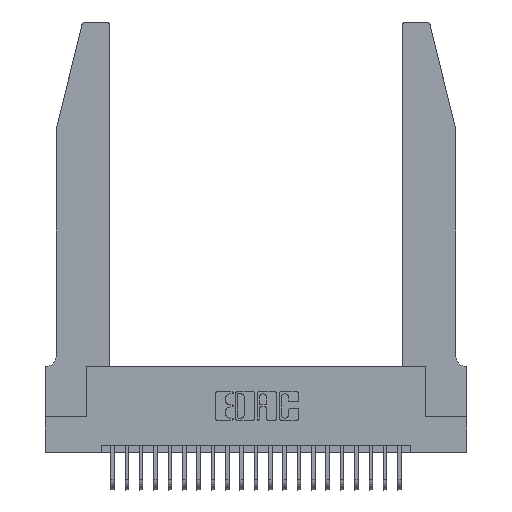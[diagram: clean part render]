
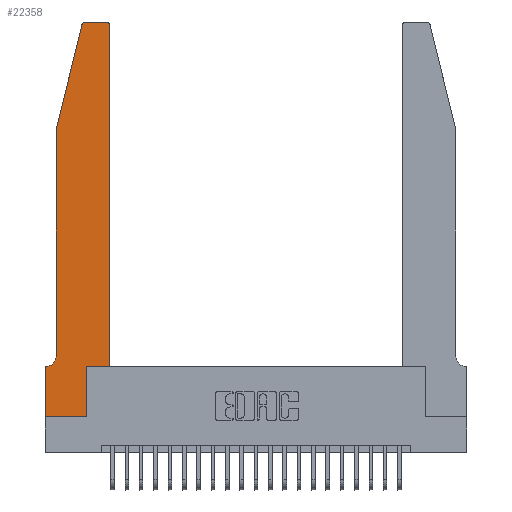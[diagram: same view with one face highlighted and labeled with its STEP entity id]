
A CAD part, top view. The second image highlights one B-rep face of the part: STEP entity #22358.
In plain terms, the highlighted planar face has unit normal (0, 0, 1).
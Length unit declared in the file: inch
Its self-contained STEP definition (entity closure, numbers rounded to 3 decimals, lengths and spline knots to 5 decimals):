
#276 = CARTESIAN_POINT ( 'NONE',  ( 0.4505, 2.72, 0.37 ) ) ;
#398 = DIRECTION ( 'NONE',  ( 1., 0., 0. ) ) ;
#477 = VERTEX_POINT ( 'NONE', #276 ) ;
#687 = AXIS2_PLACEMENT_3D ( 'NONE', #13670, #1573, #15613 ) ;
#795 = LINE ( 'NONE', #8910, #11031 ) ;
#949 = ORIENTED_EDGE ( 'NONE', *, *, #25174, .T. ) ;
#1255 = DIRECTION ( 'NONE',  ( 0., 1., 0. ) ) ;
#1522 = VECTOR ( 'NONE', #4026, 39.37008 ) ;
#1573 = DIRECTION ( 'NONE',  ( 0., 0., 1. ) ) ;
#1868 = VERTEX_POINT ( 'NONE', #6498 ) ;
#1920 = VERTEX_POINT ( 'NONE', #20154 ) ;
#1921 = CARTESIAN_POINT ( 'NONE',  ( 0.0755, 2., 0.37 ) ) ;
#2319 = AXIS2_PLACEMENT_3D ( 'NONE', #24216, #12634, #398 ) ;
#2850 = CIRCLE ( 'NONE', #23031, 0.07 ) ;
#3149 = CIRCLE ( 'NONE', #12000, 0.03 ) ;
#3510 = CARTESIAN_POINT ( 'NONE',  ( 0.2865, 0., 0.37 ) ) ;
#3579 = CARTESIAN_POINT ( 'NONE',  ( 0.0055, 0.42, 0.37 ) ) ;
#3863 = DIRECTION ( 'NONE',  ( 1., 0., 0. ) ) ;
#4026 = DIRECTION ( 'NONE',  ( 1., 0., 0. ) ) ;
#4097 = VERTEX_POINT ( 'NONE', #22387 ) ;
#4926 = ORIENTED_EDGE ( 'NONE', *, *, #16400, .T. ) ;
#5160 = VERTEX_POINT ( 'NONE', #10495 ) ;
#5360 = CARTESIAN_POINT ( 'NONE',  ( 0.2605, 2.75, 0.37 ) ) ;
#5563 = ORIENTED_EDGE ( 'NONE', *, *, #16069, .T. ) ;
#5650 = DIRECTION ( 'NONE',  ( -1., 0., 0. ) ) ;
#6498 = CARTESIAN_POINT ( 'NONE',  ( 0.25487, 2.72718, 0.37 ) ) ;
#6994 = LINE ( 'NONE', #19590, #16216 ) ;
#7205 = CARTESIAN_POINT ( 'NONE',  ( 0., 0., 0.37 ) ) ;
#7231 = VECTOR ( 'NONE', #9652, 39.37008 ) ;
#7433 = DIRECTION ( 'NONE',  ( -1., 0., 0. ) ) ;
#7659 = CARTESIAN_POINT ( 'NONE',  ( 0.2865, 0.35, 0.37 ) ) ;
#7938 = CARTESIAN_POINT ( 'NONE',  ( 0., 0., 0.37 ) ) ;
#7959 = VERTEX_POINT ( 'NONE', #14948 ) ;
#8149 = VERTEX_POINT ( 'NONE', #17433 ) ;
#8910 = CARTESIAN_POINT ( 'NONE',  ( 0.0755, 2., 0.37 ) ) ;
#8956 = LINE ( 'NONE', #13859, #18140 ) ;
#9561 = EDGE_CURVE ( 'NONE', #1920, #19440, #24381, .T. ) ;
#9652 = DIRECTION ( 'NONE',  ( 0., 1., 0. ) ) ;
#9710 = VECTOR ( 'NONE', #1255, 39.37008 ) ;
#9889 = DIRECTION ( 'NONE',  ( -1., 0., 0. ) ) ;
#10101 = VECTOR ( 'NONE', #19632, 39.37008 ) ;
#10132 = EDGE_LOOP ( 'NONE', ( #23525, #24363, #21272, #4926, #16394, #23688, #21248, #5563, #949, #20915, #19216, #16464 ) ) ;
#10495 = CARTESIAN_POINT ( 'NONE',  ( 0.0755, 0.42, 0.37 ) ) ;
#10695 = EDGE_CURVE ( 'NONE', #8149, #17127, #20692, .T. ) ;
#10889 = CARTESIAN_POINT ( 'NONE',  ( 0.4205, 2.72, 0.37 ) ) ;
#10891 = DIRECTION ( 'NONE',  ( 0., -1., 0. ) ) ;
#10953 = VECTOR ( 'NONE', #7433, 39.37008 ) ;
#11031 = VECTOR ( 'NONE', #10891, 39.37008 ) ;
#11214 = EDGE_CURVE ( 'NONE', #15154, #477, #14879, .T. ) ;
#11569 = EDGE_CURVE ( 'NONE', #17127, #1868, #17948, .T. ) ;
#12000 = AXIS2_PLACEMENT_3D ( 'NONE', #10889, #24470, #12870 ) ;
#12634 = DIRECTION ( 'NONE',  ( 0., 0., 1. ) ) ;
#12870 = DIRECTION ( 'NONE',  ( 1., 0., 0. ) ) ;
#13045 = VERTEX_POINT ( 'NONE', #3510 ) ;
#13189 = VERTEX_POINT ( 'NONE', #1921 ) ;
#13670 = CARTESIAN_POINT ( 'NONE',  ( 0., 0.35, 0.37 ) ) ;
#13804 = LINE ( 'NONE', #15768, #23543 ) ;
#13859 = CARTESIAN_POINT ( 'NONE',  ( 0.0755, 2., 0.37 ) ) ;
#14879 = LINE ( 'NONE', #23084, #9710 ) ;
#14927 = EDGE_CURVE ( 'NONE', #1868, #13189, #8956, .T. ) ;
#14948 = CARTESIAN_POINT ( 'NONE',  ( 0.0055, 0.35, 0.37 ) ) ;
#15154 = VERTEX_POINT ( 'NONE', #20471 ) ;
#15613 = DIRECTION ( 'NONE',  ( 1., 0., 0. ) ) ;
#15768 = CARTESIAN_POINT ( 'NONE',  ( 0., 0., 0.37 ) ) ;
#15823 = DIRECTION ( 'NONE',  ( -0.239, -0.971, 0. ) ) ;
#15932 = CARTESIAN_POINT ( 'NONE',  ( 0.4505, 0.35, 0.37 ) ) ;
#16069 = EDGE_CURVE ( 'NONE', #19440, #13045, #13804, .T. ) ;
#16216 = VECTOR ( 'NONE', #9889, 39.37008 ) ;
#16340 = CARTESIAN_POINT ( 'NONE',  ( 0.284, 2.75, 0.37 ) ) ;
#16394 = ORIENTED_EDGE ( 'NONE', *, *, #22010, .T. ) ;
#16400 = EDGE_CURVE ( 'NONE', #13189, #5160, #795, .T. ) ;
#16464 = ORIENTED_EDGE ( 'NONE', *, *, #23301, .T. ) ;
#17127 = VERTEX_POINT ( 'NONE', #16340 ) ;
#17433 = CARTESIAN_POINT ( 'NONE',  ( 0.4205, 2.75, 0.37 ) ) ;
#17469 = DIRECTION ( 'NONE',  ( 0., 0., -1. ) ) ;
#17948 = CIRCLE ( 'NONE', #2319, 0.03 ) ;
#18140 = VECTOR ( 'NONE', #15823, 39.37008 ) ;
#19216 = ORIENTED_EDGE ( 'NONE', *, *, #11214, .T. ) ;
#19440 = VERTEX_POINT ( 'NONE', #7205 ) ;
#19590 = CARTESIAN_POINT ( 'NONE',  ( 0.0755, 0.35, 0.37 ) ) ;
#19632 = DIRECTION ( 'NONE',  ( 0., -1., 0. ) ) ;
#20154 = CARTESIAN_POINT ( 'NONE',  ( 0., 0.35, 0.37 ) ) ;
#20471 = CARTESIAN_POINT ( 'NONE',  ( 0.4505, 0.35, 0.37 ) ) ;
#20692 = LINE ( 'NONE', #5360, #10953 ) ;
#20915 = ORIENTED_EDGE ( 'NONE', *, *, #22157, .T. ) ;
#21248 = ORIENTED_EDGE ( 'NONE', *, *, #9561, .T. ) ;
#21272 = ORIENTED_EDGE ( 'NONE', *, *, #14927, .T. ) ;
#21406 = PLANE ( 'NONE',  #687 ) ;
#22010 = EDGE_CURVE ( 'NONE', #5160, #7959, #2850, .T. ) ;
#22157 = EDGE_CURVE ( 'NONE', #4097, #15154, #24730, .T. ) ;
#22244 = LINE ( 'NONE', #7659, #7231 ) ;
#22358 = ADVANCED_FACE ( 'NONE', ( #25013 ), #21406, .T. ) ;
#22387 = CARTESIAN_POINT ( 'NONE',  ( 0.2865, 0.35, 0.37 ) ) ;
#22961 = EDGE_CURVE ( 'NONE', #7959, #1920, #6994, .T. ) ;
#23031 = AXIS2_PLACEMENT_3D ( 'NONE', #3579, #17469, #5650 ) ;
#23084 = CARTESIAN_POINT ( 'NONE',  ( 0.4505, 0.35, 0.37 ) ) ;
#23301 = EDGE_CURVE ( 'NONE', #477, #8149, #3149, .T. ) ;
#23525 = ORIENTED_EDGE ( 'NONE', *, *, #10695, .T. ) ;
#23543 = VECTOR ( 'NONE', #3863, 39.37008 ) ;
#23688 = ORIENTED_EDGE ( 'NONE', *, *, #22961, .T. ) ;
#24216 = CARTESIAN_POINT ( 'NONE',  ( 0.284, 2.72, 0.37 ) ) ;
#24363 = ORIENTED_EDGE ( 'NONE', *, *, #11569, .T. ) ;
#24381 = LINE ( 'NONE', #7938, #10101 ) ;
#24470 = DIRECTION ( 'NONE',  ( 0., 0., 1. ) ) ;
#24730 = LINE ( 'NONE', #15932, #1522 ) ;
#25013 = FACE_OUTER_BOUND ( 'NONE', #10132, .T. ) ;
#25174 = EDGE_CURVE ( 'NONE', #13045, #4097, #22244, .T. ) ;
